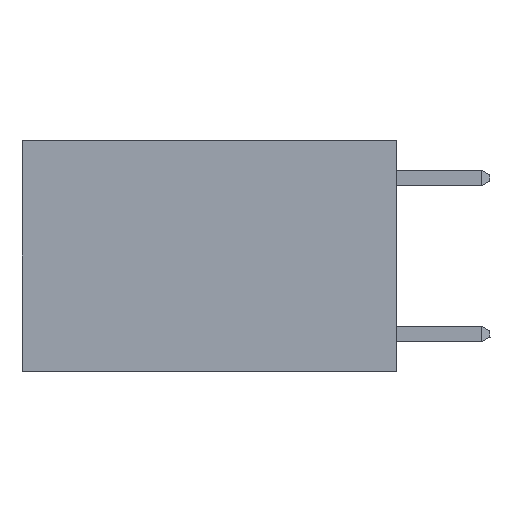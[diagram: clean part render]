
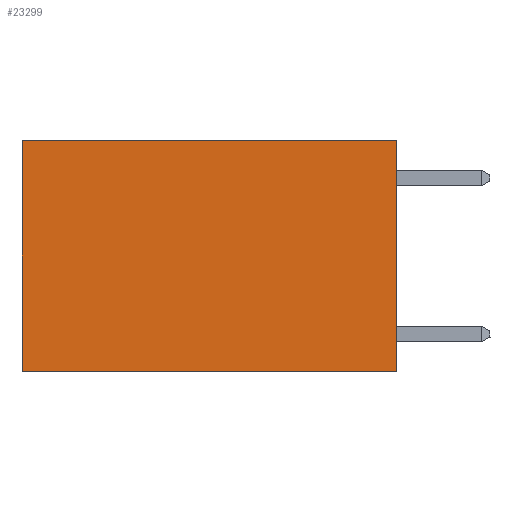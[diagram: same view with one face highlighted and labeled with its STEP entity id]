
A CAD part, left-side view. The second image highlights one B-rep face of the part: STEP entity #23299.
In plain terms, the highlighted planar face has unit normal (-1, 0, 0).
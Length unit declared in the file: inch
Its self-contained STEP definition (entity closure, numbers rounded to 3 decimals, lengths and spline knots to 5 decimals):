
#203 = LINE ( 'NONE', #16711, #887 ) ;
#241 = EDGE_LOOP ( 'NONE', ( #20678, #3479, #2902, #8577 ) ) ;
#887 = VECTOR ( 'NONE', #20914, 39.37008 ) ;
#1880 = CARTESIAN_POINT ( 'NONE',  ( 0.2625, 0.6, 0. ) ) ;
#2410 = CARTESIAN_POINT ( 'NONE',  ( 0.2625, 0., 0. ) ) ;
#2902 = ORIENTED_EDGE ( 'NONE', *, *, #13258, .F. ) ;
#3479 = ORIENTED_EDGE ( 'NONE', *, *, #20272, .F. ) ;
#4616 = DIRECTION ( 'NONE',  ( 0., 0., -1. ) ) ;
#5745 = VERTEX_POINT ( 'NONE', #15685 ) ;
#6047 = VERTEX_POINT ( 'NONE', #16971 ) ;
#6701 = PLANE ( 'NONE',  #17402 ) ;
#8577 = ORIENTED_EDGE ( 'NONE', *, *, #9157, .T. ) ;
#9039 = VECTOR ( 'NONE', #16805, 39.37008 ) ;
#9157 = EDGE_CURVE ( 'NONE', #16482, #12472, #25418, .T. ) ;
#9454 = FACE_OUTER_BOUND ( 'NONE', #241, .T. ) ;
#12472 = VERTEX_POINT ( 'NONE', #1880 ) ;
#12605 = DIRECTION ( 'NONE',  ( 0., 1., 0. ) ) ;
#13258 = EDGE_CURVE ( 'NONE', #16482, #6047, #14534, .T. ) ;
#13781 = VECTOR ( 'NONE', #12605, 39.37008 ) ;
#13865 = VECTOR ( 'NONE', #23243, 39.37008 ) ;
#14534 = LINE ( 'NONE', #21203, #13865 ) ;
#14678 = CARTESIAN_POINT ( 'NONE',  ( 0.2625, 0., -0.37 ) ) ;
#15685 = CARTESIAN_POINT ( 'NONE',  ( 0.2625, 0.6, -0.37 ) ) ;
#16482 = VERTEX_POINT ( 'NONE', #23688 ) ;
#16711 = CARTESIAN_POINT ( 'NONE',  ( 0.2625, 0.6, 0. ) ) ;
#16805 = DIRECTION ( 'NONE',  ( 0., 1., 0. ) ) ;
#16971 = CARTESIAN_POINT ( 'NONE',  ( 0.2625, 0., -0.37 ) ) ;
#17258 = DIRECTION ( 'NONE',  ( 1., 0., 0. ) ) ;
#17402 = AXIS2_PLACEMENT_3D ( 'NONE', #2410, #17258, #4616 ) ;
#20185 = LINE ( 'NONE', #14678, #9039 ) ;
#20272 = EDGE_CURVE ( 'NONE', #6047, #5745, #20185, .T. ) ;
#20678 = ORIENTED_EDGE ( 'NONE', *, *, #25218, .T. ) ;
#20914 = DIRECTION ( 'NONE',  ( 0., 0., -1. ) ) ;
#21203 = CARTESIAN_POINT ( 'NONE',  ( 0.2625, 0., 0. ) ) ;
#22996 = CARTESIAN_POINT ( 'NONE',  ( 0.2625, 0., 0. ) ) ;
#23243 = DIRECTION ( 'NONE',  ( 0., 0., -1. ) ) ;
#23299 = ADVANCED_FACE ( 'NONE', ( #9454 ), #6701, .F. ) ;
#23688 = CARTESIAN_POINT ( 'NONE',  ( 0.2625, 0., 0. ) ) ;
#25218 = EDGE_CURVE ( 'NONE', #12472, #5745, #203, .T. ) ;
#25418 = LINE ( 'NONE', #22996, #13781 ) ;
